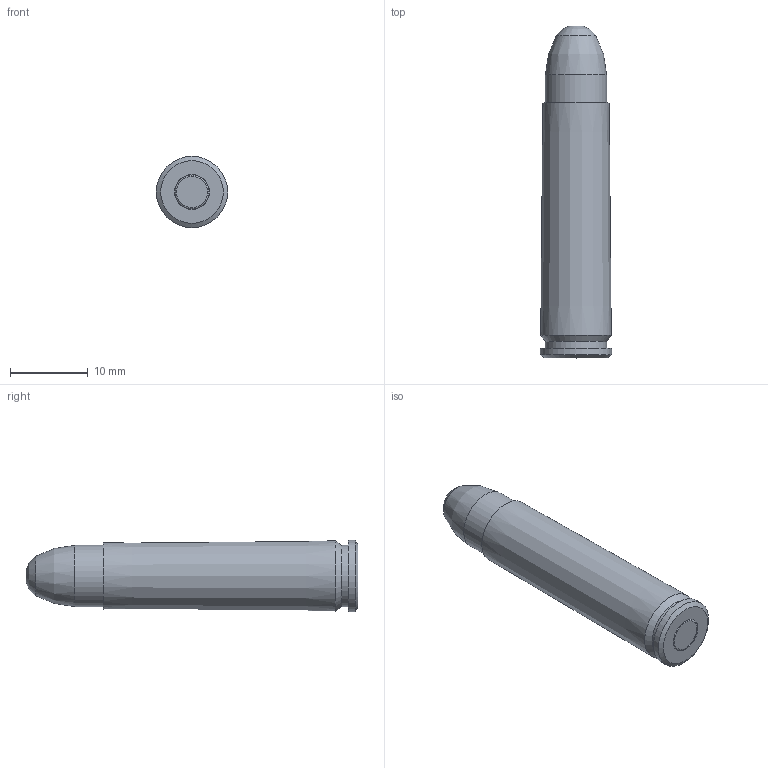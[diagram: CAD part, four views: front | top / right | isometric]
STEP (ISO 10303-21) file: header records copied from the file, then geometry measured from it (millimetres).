
FILE_DESCRIPTION((''),'2;1');
FILE_NAME('30 M1 CARBINE.stp','2012-12-03T08:26:18',('agarrett'),(''),'Autodesk Inventor 2012','Autodesk Inventor 2012','');
FILE_SCHEMA(('AUTOMOTIVE_DESIGN { 1 0 10303 214 1 1 1 1 }'));
Length unit declared in the file: inch
Products named in the file (4): iLogic Cartridge; Rimless Straight; iLogic RN Bullet; PRIMER
Assembly tree (3 placements, depth 2):
  iLogic Cartridge
    Rimless Straight
    iLogic RN Bullet
    PRIMER
Bounding box: 9.14 x 42.67 x 9.14 mm (x, y, z)
Volume: 1146 mm3; surface area: 2391.7 mm2
Topology: 3 solids, 3 shells, 27 faces, 42 edges, 25 vertices
Faces by surface type: plane 10, cylinder 7, cone 4, torus 4, bspline 2
Full cylindrical faces by diameter (mm): 1.778 x1, 4.191 x1, 4.445 x2, 7.851 x1, 7.869 x1, 9.139 x1
Entity records: 718 total; most frequent: CARTESIAN_POINT 136, DIRECTION 114, AXIS2_PLACEMENT_3D 57, ORIENTED_EDGE 50, EDGE_LOOP 50, FACE_OUTER_BOUND 27, ADVANCED_FACE 27, VERTEX_POINT 25
